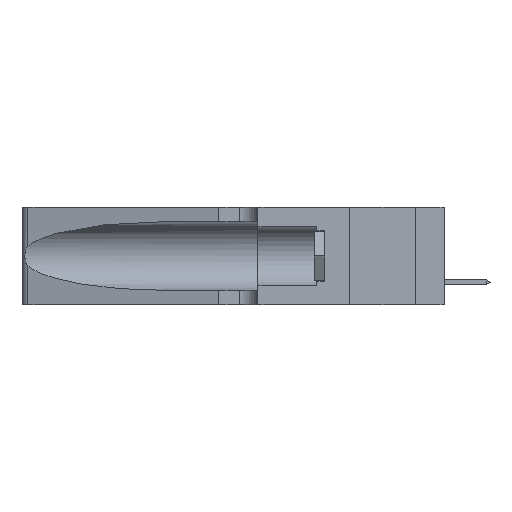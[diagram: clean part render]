
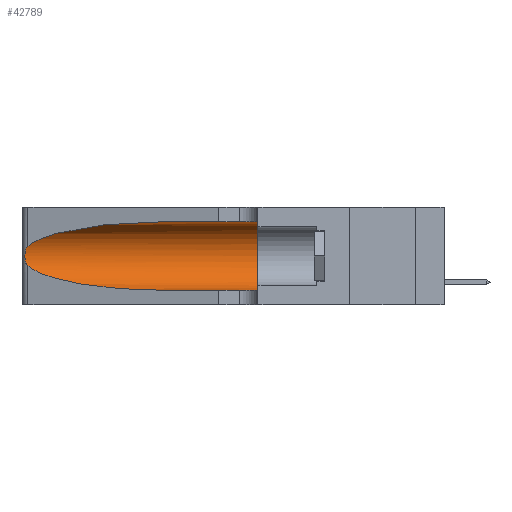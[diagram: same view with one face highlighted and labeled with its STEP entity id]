
A CAD part, left-side view. The second image highlights one B-rep face of the part: STEP entity #42789.
In plain terms, the highlighted cylindrical face has radius 3.308 mm (diameter 6.617 mm), a partial arc.
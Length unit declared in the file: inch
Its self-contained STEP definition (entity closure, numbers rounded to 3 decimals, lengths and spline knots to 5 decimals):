
#1757 = VERTEX_POINT ( 'NONE', #34826 ) ;
#2592 = CARTESIAN_POINT ( 'NONE',  ( 0.2373, 1.15595, 0.28018 ) ) ;
#2735 = CARTESIAN_POINT ( 'NONE',  ( 0.18966, 0.96281, 0.31525 ) ) ;
#3058 = EDGE_CURVE ( 'NONE', #32785, #42662, #6229, .T. ) ;
#3114 = VECTOR ( 'NONE', #21853, 39.37008 ) ;
#3532 = CARTESIAN_POINT ( 'NONE',  ( 0.25487, 1.22718, 0.22369 ) ) ;
#3700 = DIRECTION ( 'NONE',  ( 0., -1., 0. ) ) ;
#5446 = CARTESIAN_POINT ( 'NONE',  ( 0.25854, 1.2359, 0.20912 ) ) ;
#5589 = CARTESIAN_POINT ( 'NONE',  ( 0.26017, 1.23833, 0.17102 ) ) ;
#6229 = B_SPLINE_CURVE_WITH_KNOTS ( 'NONE', 3,
 ( #30467, #12034, #36975, #12663, #5446, #15566, #8949, #30140, #5589, #37130, #37453, #22726, #43899, #40672 ),
 .UNSPECIFIED., .F., .F.,
 ( 4, 2, 2, 2, 2, 2, 4 ),
 ( 0., 0.00027, 0.00053, 0.00107, 0.0016, 0.00187, 0.00214 ),
 .UNSPECIFIED. ) ;
#6925 = CARTESIAN_POINT ( 'NONE',  ( 0.1305, 0.35, 0.05475 ) ) ;
#8496 = VERTEX_POINT ( 'NONE', #6925 ) ;
#8949 = CARTESIAN_POINT ( 'NONE',  ( 0.26075, 1.23896, 0.19203 ) ) ;
#9711 = FACE_OUTER_BOUND ( 'NONE', #44212, .T. ) ;
#9742 = CARTESIAN_POINT ( 'NONE',  ( 0.2373, 1.15595, 0.08982 ) ) ;
#10218 = AXIS2_PLACEMENT_3D ( 'NONE', #19541, #29918, #36751 ) ;
#10564 = EDGE_CURVE ( 'NONE', #42662, #35607, #27439, .T. ) ;
#11142 = CARTESIAN_POINT ( 'NONE',  ( 0.1305, 1.61858, 0.05475 ) ) ;
#11943 = EDGE_CURVE ( 'NONE', #35607, #8496, #42713, .T. ) ;
#12034 = CARTESIAN_POINT ( 'NONE',  ( 0.25555, 1.22994, 0.2215 ) ) ;
#12399 = DIRECTION ( 'NONE',  ( 0., -1., 0. ) ) ;
#12425 = CYLINDRICAL_SURFACE ( 'NONE', #22063, 0.13025 ) ;
#12663 = CARTESIAN_POINT ( 'NONE',  ( 0.25787, 1.23484, 0.2124 ) ) ;
#13437 = VECTOR ( 'NONE', #12399, 39.37008 ) ;
#14182 = DIRECTION ( 'NONE',  ( 0., 0., -1. ) ) ;
#15566 = CARTESIAN_POINT ( 'NONE',  ( 0.26018, 1.23835, 0.19895 ) ) ;
#17652 = CARTESIAN_POINT ( 'NONE',  ( 0.1305, 1.61858, 0.31525 ) ) ;
#19541 = CARTESIAN_POINT ( 'NONE',  ( 0.1305, 0.35, 0.185 ) ) ;
#21009 = CIRCLE ( 'NONE', #10218, 0.13025 ) ;
#21853 = DIRECTION ( 'NONE',  ( 0., -1., 0. ) ) ;
#22063 = AXIS2_PLACEMENT_3D ( 'NONE', #35841, #3700, #14182 ) ;
#22669 = EDGE_CURVE ( 'NONE', #1757, #8496, #21009, .T. ) ;
#22726 = CARTESIAN_POINT ( 'NONE',  ( 0.25639, 1.23186, 0.15144 ) ) ;
#23749 = CARTESIAN_POINT ( 'NONE',  ( 0.1305, 0.72297, 0.31525 ) ) ;
#24039 = CARTESIAN_POINT ( 'NONE',  ( 0.25487, 1.22718, 0.22369 ) ) ;
#25194 = ORIENTED_EDGE ( 'NONE', *, *, #11943, .T. ) ;
#27439 =( BOUNDED_CURVE ( )  B_SPLINE_CURVE ( 3, ( #30918, #9742, #38060, #45136 ),
 .UNSPECIFIED., .F., .T. ) 
 B_SPLINE_CURVE_WITH_KNOTS ( ( 4, 4 ),
 ( 3.44316, 4.71239 ),
 .UNSPECIFIED. ) 
 CURVE ( )  GEOMETRIC_REPRESENTATION_ITEM ( )  RATIONAL_B_SPLINE_CURVE ( ( 1., 0.87, 0.87, 1. ) ) 
 REPRESENTATION_ITEM ( '' )  );
#27506 = ORIENTED_EDGE ( 'NONE', *, *, #22669, .F. ) ;
#28410 = CARTESIAN_POINT ( 'NONE',  ( 0.25487, 1.22718, 0.14631 ) ) ;
#29918 = DIRECTION ( 'NONE',  ( 0., 1., 0. ) ) ;
#30105 = CARTESIAN_POINT ( 'NONE',  ( 0.1305, 0.72297, 0.05475 ) ) ;
#30134 = CARTESIAN_POINT ( 'NONE',  ( 0.1305, 0.72297, 0.31525 ) ) ;
#30140 = CARTESIAN_POINT ( 'NONE',  ( 0.26075, 1.23896, 0.178 ) ) ;
#30467 = CARTESIAN_POINT ( 'NONE',  ( 0.25487, 1.22718, 0.22369 ) ) ;
#30918 = CARTESIAN_POINT ( 'NONE',  ( 0.25487, 1.22718, 0.14631 ) ) ;
#32456 = VERTEX_POINT ( 'NONE', #30134 ) ;
#32785 = VERTEX_POINT ( 'NONE', #3532 ) ;
#34590 = EDGE_CURVE ( 'NONE', #32456, #32785, #40491, .T. ) ;
#34826 = CARTESIAN_POINT ( 'NONE',  ( 0.1305, 0.35, 0.31525 ) ) ;
#35607 = VERTEX_POINT ( 'NONE', #30105 ) ;
#35841 = CARTESIAN_POINT ( 'NONE',  ( 0.1305, 1.61858, 0.185 ) ) ;
#36066 = EDGE_CURVE ( 'NONE', #32456, #1757, #38022, .T. ) ;
#36751 = DIRECTION ( 'NONE',  ( 0., 0., 1. ) ) ;
#36975 = CARTESIAN_POINT ( 'NONE',  ( 0.25639, 1.23184, 0.21858 ) ) ;
#37130 = CARTESIAN_POINT ( 'NONE',  ( 0.25856, 1.23593, 0.16098 ) ) ;
#37453 = CARTESIAN_POINT ( 'NONE',  ( 0.25789, 1.23486, 0.15765 ) ) ;
#38022 = LINE ( 'NONE', #17652, #3114 ) ;
#38060 = CARTESIAN_POINT ( 'NONE',  ( 0.18966, 0.96281, 0.05475 ) ) ;
#39675 = ORIENTED_EDGE ( 'NONE', *, *, #36066, .F. ) ;
#40491 =( BOUNDED_CURVE ( )  B_SPLINE_CURVE ( 3, ( #23749, #2735, #2592, #24039 ),
 .UNSPECIFIED., .F., .F. ) 
 B_SPLINE_CURVE_WITH_KNOTS ( ( 4, 4 ),
 ( 1.5708, 2.84003 ),
 .UNSPECIFIED. ) 
 CURVE ( )  GEOMETRIC_REPRESENTATION_ITEM ( )  RATIONAL_B_SPLINE_CURVE ( ( 1., 0.87, 0.87, 1. ) ) 
 REPRESENTATION_ITEM ( '' )  );
#40672 = CARTESIAN_POINT ( 'NONE',  ( 0.25487, 1.22718, 0.14631 ) ) ;
#41969 = ORIENTED_EDGE ( 'NONE', *, *, #3058, .T. ) ;
#42084 = ORIENTED_EDGE ( 'NONE', *, *, #34590, .T. ) ;
#42662 = VERTEX_POINT ( 'NONE', #28410 ) ;
#42713 = LINE ( 'NONE', #11142, #13437 ) ;
#42789 = ADVANCED_FACE ( 'NONE', ( #9711 ), #12425, .F. ) ;
#43899 = CARTESIAN_POINT ( 'NONE',  ( 0.25555, 1.22993, 0.14849 ) ) ;
#44085 = ORIENTED_EDGE ( 'NONE', *, *, #10564, .T. ) ;
#44212 = EDGE_LOOP ( 'NONE', ( #42084, #41969, #44085, #25194, #27506, #39675 ) ) ;
#45136 = CARTESIAN_POINT ( 'NONE',  ( 0.1305, 0.72297, 0.05475 ) ) ;
